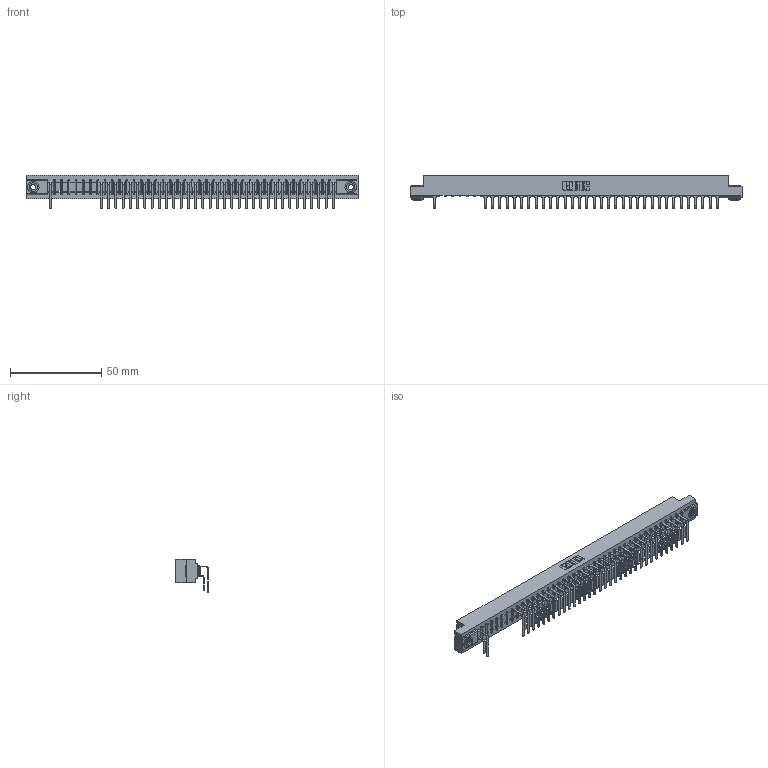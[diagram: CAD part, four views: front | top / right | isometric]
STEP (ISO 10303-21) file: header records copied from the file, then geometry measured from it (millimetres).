
FILE_DESCRIPTION (( 'STEP AP203' ), '1' );
FILE_NAME ('307-040-559-103.STEP', '2018-08-05T13:59:34', ( '' ), ( '' ), 'SwSTEP 2.0', 'SolidWorks 2016', '' );
FILE_SCHEMA (( 'CONFIG_CONTROL_DESIGN' ));
Length unit declared in the file: inch
Products named in the file (5): 345-250-002_345-250-002-102; 307-040-559-103; 307 Part_.156 Dia Mounting Holes; 307-290-001_558 559 - 1 (Single); 307-290-001_559 - 2 (Single)
Assembly tree (70 placements, depth 2):
  307-040-559-103
    307 Part_.156 Dia Mounting Holes
    307-290-001_558 559 - 1 (Single)  x33
    307-290-001_559 - 2 (Single)  x34
    345-250-002_345-250-002-102  x2
Bounding box: 181.51 x 17.69 x 18.07 mm (x, y, z)
Volume: 19418.8 mm3; surface area: 24606 mm2
Topology: 70 solids, 70 shells, 3691 faces, 10365 edges, 6706 vertices
Faces by surface type: plane 2383, cylinder 1218, sphere 82, cone 8
Entity records: 37914 total; most frequent: CARTESIAN_POINT 6242, ORIENTED_EDGE 6190, DIRECTION 6115, EDGE_CURVE 3095, LINE 2365, VECTOR 2365, VERTEX_POINT 2002, AXIS2_PLACEMENT_3D 1875
